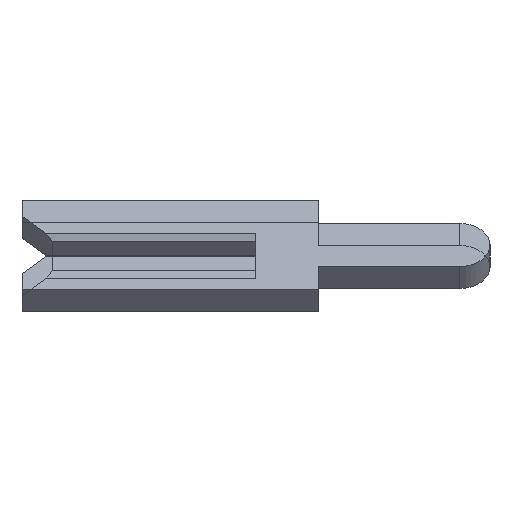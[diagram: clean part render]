
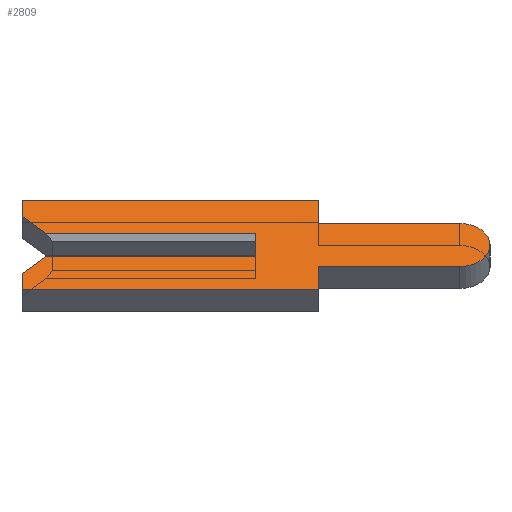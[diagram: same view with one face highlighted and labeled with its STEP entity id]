
A CAD part, left-side view. The second image highlights one B-rep face of the part: STEP entity #2809.
In plain terms, the highlighted face is planar.
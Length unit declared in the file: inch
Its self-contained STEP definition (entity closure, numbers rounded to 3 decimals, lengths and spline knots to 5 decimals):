
#24 = VECTOR ( 'NONE', #2257, 39.37008 ) ;
#116 = ORIENTED_EDGE ( 'NONE', *, *, #2890, .F. ) ;
#140 = EDGE_CURVE ( 'NONE', #1124, #1795, #364, .T. ) ;
#168 = CARTESIAN_POINT ( 'NONE',  ( -0.01, 0.15, -0.04 ) ) ;
#219 = LINE ( 'NONE', #3028, #610 ) ;
#222 = ORIENTED_EDGE ( 'NONE', *, *, #2678, .F. ) ;
#257 = AXIS2_PLACEMENT_3D ( 'NONE', #2248, #1612, #1534 ) ;
#258 = ORIENTED_EDGE ( 'NONE', *, *, #2549, .T. ) ;
#264 = FACE_OUTER_BOUND ( 'NONE', #3906, .T. ) ;
#270 = VECTOR ( 'NONE', #730, 39.37008 ) ;
#332 = CARTESIAN_POINT ( 'NONE',  ( -0.01, -0.1305, 0.0195 ) ) ;
#357 = CARTESIAN_POINT ( 'NONE',  ( -0.01, -0.04, -0.0195 ) ) ;
#364 = LINE ( 'NONE', #3921, #270 ) ;
#371 = DIRECTION ( 'NONE',  ( 1., 0., 0. ) ) ;
#420 = ORIENTED_EDGE ( 'NONE', *, *, #3275, .F. ) ;
#562 = LINE ( 'NONE', #1931, #3811 ) ;
#610 = VECTOR ( 'NONE', #2469, 39.37008 ) ;
#655 = ORIENTED_EDGE ( 'NONE', *, *, #1114, .F. ) ;
#658 = PLANE ( 'NONE',  #3035 ) ;
#686 = CARTESIAN_POINT ( 'NONE',  ( -0.01, 0.15, -0.04 ) ) ;
#730 = DIRECTION ( 'NONE',  ( 0., 0., -1. ) ) ;
#779 = VERTEX_POINT ( 'NONE', #168 ) ;
#783 = EDGE_CURVE ( 'NONE', #2175, #3012, #2313, .T. ) ;
#880 = VECTOR ( 'NONE', #1011, 39.37008 ) ;
#917 = LINE ( 'NONE', #2080, #2010 ) ;
#932 = ORIENTED_EDGE ( 'NONE', *, *, #2598, .F. ) ;
#937 = VECTOR ( 'NONE', #3469, 39.37008 ) ;
#964 = ORIENTED_EDGE ( 'NONE', *, *, #1779, .F. ) ;
#1011 = DIRECTION ( 'NONE',  ( 0., 1., 0. ) ) ;
#1026 = CARTESIAN_POINT ( 'NONE',  ( -0.01, 0.15, 0.026 ) ) ;
#1052 = EDGE_CURVE ( 'NONE', #779, #3440, #917, .T. ) ;
#1107 = DIRECTION ( 'NONE',  ( 0., -1., 0. ) ) ;
#1114 = EDGE_CURVE ( 'NONE', #3440, #3797, #3609, .T. ) ;
#1124 = VERTEX_POINT ( 'NONE', #1758 ) ;
#1240 = VERTEX_POINT ( 'NONE', #1774 ) ;
#1323 = CIRCLE ( 'NONE', #257, 0.0195 ) ;
#1426 = LINE ( 'NONE', #1856, #24 ) ;
#1525 = LINE ( 'NONE', #357, #937 ) ;
#1534 = DIRECTION ( 'NONE',  ( 0., 0., -1. ) ) ;
#1574 = LINE ( 'NONE', #686, #880 ) ;
#1612 = DIRECTION ( 'NONE',  ( 1., 0., 0. ) ) ;
#1640 = DIRECTION ( 'NONE',  ( 0., -1., 0. ) ) ;
#1758 = CARTESIAN_POINT ( 'NONE',  ( -0.01, -0.04, -0.0195 ) ) ;
#1774 = CARTESIAN_POINT ( 'NONE',  ( -0.01, 0.134, 0.01 ) ) ;
#1779 = EDGE_CURVE ( 'NONE', #3797, #2267, #219, .T. ) ;
#1795 = VERTEX_POINT ( 'NONE', #2454 ) ;
#1853 = VERTEX_POINT ( 'NONE', #3711 ) ;
#1856 = CARTESIAN_POINT ( 'NONE',  ( -0.01, -0.04, 0.0195 ) ) ;
#1880 = ORIENTED_EDGE ( 'NONE', *, *, #783, .F. ) ;
#1919 = CARTESIAN_POINT ( 'NONE',  ( -0.01, -0.04, 0.04 ) ) ;
#1931 = CARTESIAN_POINT ( 'NONE',  ( -0.01, 0.1305, 0.0065 ) ) ;
#1948 = CARTESIAN_POINT ( 'NONE',  ( -0.01, -0.1305, 0. ) ) ;
#2010 = VECTOR ( 'NONE', #3652, 39.37008 ) ;
#2021 = CARTESIAN_POINT ( 'NONE',  ( -0.01, 0.15, -0.026 ) ) ;
#2061 = LINE ( 'NONE', #2288, #3111 ) ;
#2080 = CARTESIAN_POINT ( 'NONE',  ( -0.01, 0.15, -0.026 ) ) ;
#2105 = EDGE_CURVE ( 'NONE', #2267, #2901, #2508, .T. ) ;
#2141 = DIRECTION ( 'NONE',  ( 0., 0., 1. ) ) ;
#2175 = VERTEX_POINT ( 'NONE', #3446 ) ;
#2248 = CARTESIAN_POINT ( 'NONE',  ( -0.01, -0.1305, 0. ) ) ;
#2257 = DIRECTION ( 'NONE',  ( 0., -1., 0. ) ) ;
#2267 = VERTEX_POINT ( 'NONE', #2746 ) ;
#2274 = DIRECTION ( 'NONE',  ( 0., 0., -1. ) ) ;
#2275 = LINE ( 'NONE', #1026, #2377 ) ;
#2288 = CARTESIAN_POINT ( 'NONE',  ( -0.01, 0.15, 0.01 ) ) ;
#2313 = LINE ( 'NONE', #3322, #2957 ) ;
#2377 = VECTOR ( 'NONE', #3263, 39.37008 ) ;
#2454 = CARTESIAN_POINT ( 'NONE',  ( -0.01, -0.04, -0.04 ) ) ;
#2469 = DIRECTION ( 'NONE',  ( 0., -1., 0. ) ) ;
#2475 = VECTOR ( 'NONE', #3129, 39.37008 ) ;
#2508 = LINE ( 'NONE', #3738, #3770 ) ;
#2549 = EDGE_CURVE ( 'NONE', #1240, #2901, #2061, .T. ) ;
#2561 = ORIENTED_EDGE ( 'NONE', *, *, #3930, .F. ) ;
#2563 = CARTESIAN_POINT ( 'NONE',  ( -0.01, -0.04, 0.04 ) ) ;
#2598 = EDGE_CURVE ( 'NONE', #2764, #3422, #1323, .T. ) ;
#2678 = EDGE_CURVE ( 'NONE', #1240, #1853, #562, .T. ) ;
#2746 = CARTESIAN_POINT ( 'NONE',  ( -0.01, 0., -0.01 ) ) ;
#2764 = VERTEX_POINT ( 'NONE', #332 ) ;
#2809 = ADVANCED_FACE ( 'NONE', ( #264 ), #658, .F. ) ;
#2890 = EDGE_CURVE ( 'NONE', #3012, #3426, #3324, .T. ) ;
#2892 = ORIENTED_EDGE ( 'NONE', *, *, #2948, .F. ) ;
#2901 = VERTEX_POINT ( 'NONE', #3564 ) ;
#2948 = EDGE_CURVE ( 'NONE', #3422, #1124, #1525, .T. ) ;
#2957 = VECTOR ( 'NONE', #1107, 39.37008 ) ;
#3012 = VERTEX_POINT ( 'NONE', #2563 ) ;
#3028 = CARTESIAN_POINT ( 'NONE',  ( -0.01, -0.1305, -0.01 ) ) ;
#3035 = AXIS2_PLACEMENT_3D ( 'NONE', #1948, #371, #2274 ) ;
#3111 = VECTOR ( 'NONE', #1640, 39.37008 ) ;
#3129 = DIRECTION ( 'NONE',  ( 0., 0., -1. ) ) ;
#3141 = CARTESIAN_POINT ( 'NONE',  ( -0.01, -0.04, 0.0195 ) ) ;
#3239 = ORIENTED_EDGE ( 'NONE', *, *, #2105, .F. ) ;
#3262 = VECTOR ( 'NONE', #3681, 39.37008 ) ;
#3263 = DIRECTION ( 'NONE',  ( 0., 0., 1. ) ) ;
#3275 = EDGE_CURVE ( 'NONE', #3426, #2764, #1426, .T. ) ;
#3279 = CARTESIAN_POINT ( 'NONE',  ( -0.01, 0.134, -0.01 ) ) ;
#3322 = CARTESIAN_POINT ( 'NONE',  ( -0.01, 0.15, 0.04 ) ) ;
#3324 = LINE ( 'NONE', #1919, #2475 ) ;
#3339 = CARTESIAN_POINT ( 'NONE',  ( -0.01, 0.1305, -0.0065 ) ) ;
#3422 = VERTEX_POINT ( 'NONE', #3902 ) ;
#3426 = VERTEX_POINT ( 'NONE', #3141 ) ;
#3440 = VERTEX_POINT ( 'NONE', #2021 ) ;
#3446 = CARTESIAN_POINT ( 'NONE',  ( -0.01, 0.15, 0.04 ) ) ;
#3469 = DIRECTION ( 'NONE',  ( 0., 1., 0. ) ) ;
#3526 = ORIENTED_EDGE ( 'NONE', *, *, #3635, .F. ) ;
#3564 = CARTESIAN_POINT ( 'NONE',  ( -0.01, 0., 0.01 ) ) ;
#3568 = ORIENTED_EDGE ( 'NONE', *, *, #140, .F. ) ;
#3609 = LINE ( 'NONE', #3339, #3262 ) ;
#3635 = EDGE_CURVE ( 'NONE', #1795, #779, #1574, .T. ) ;
#3652 = DIRECTION ( 'NONE',  ( 0., 0., 1. ) ) ;
#3681 = DIRECTION ( 'NONE',  ( 0., -0.707, 0.707 ) ) ;
#3711 = CARTESIAN_POINT ( 'NONE',  ( -0.01, 0.15, 0.026 ) ) ;
#3738 = CARTESIAN_POINT ( 'NONE',  ( -0.01, 0., 0.0065 ) ) ;
#3770 = VECTOR ( 'NONE', #2141, 39.37008 ) ;
#3794 = DIRECTION ( 'NONE',  ( 0., 0.707, 0.707 ) ) ;
#3797 = VERTEX_POINT ( 'NONE', #3279 ) ;
#3811 = VECTOR ( 'NONE', #3794, 39.37008 ) ;
#3902 = CARTESIAN_POINT ( 'NONE',  ( -0.01, -0.1305, -0.0195 ) ) ;
#3906 = EDGE_LOOP ( 'NONE', ( #258, #3239, #964, #655, #3927, #3526, #3568, #2892, #932, #420, #116, #1880, #2561, #222 ) ) ;
#3921 = CARTESIAN_POINT ( 'NONE',  ( -0.01, -0.04, -0.04 ) ) ;
#3927 = ORIENTED_EDGE ( 'NONE', *, *, #1052, .F. ) ;
#3930 = EDGE_CURVE ( 'NONE', #1853, #2175, #2275, .T. ) ;
